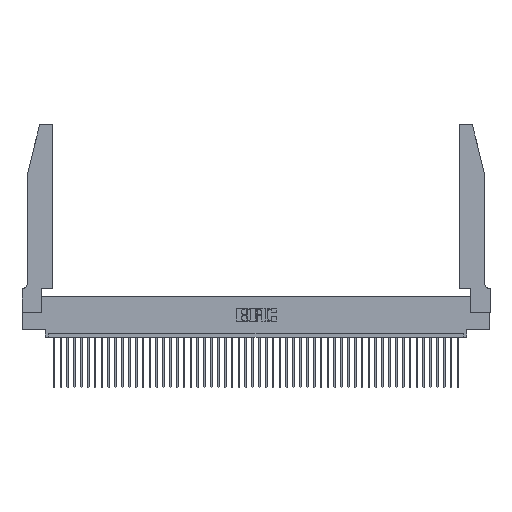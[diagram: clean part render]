
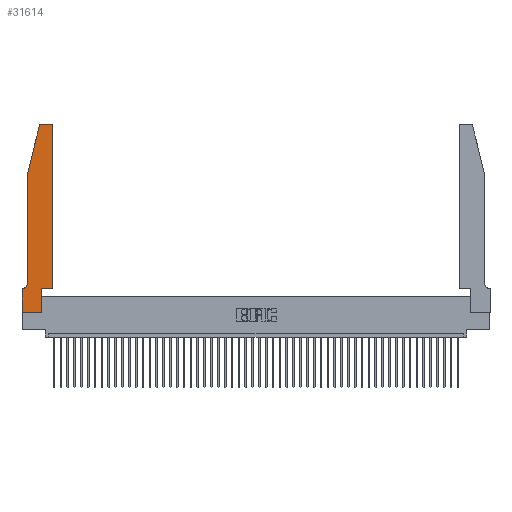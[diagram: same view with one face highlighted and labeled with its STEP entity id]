
A CAD part, top view. The second image highlights one B-rep face of the part: STEP entity #31614.
In plain terms, the highlighted planar face has unit normal (0, 0, 1).
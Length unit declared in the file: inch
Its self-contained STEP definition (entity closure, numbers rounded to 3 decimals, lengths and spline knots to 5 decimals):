
#849 = LINE ( 'NONE', #23890, #14673 ) ;
#1057 = VERTEX_POINT ( 'NONE', #4932 ) ;
#1061 = ORIENTED_EDGE ( 'NONE', *, *, #10899, .T. ) ;
#1117 = CARTESIAN_POINT ( 'NONE',  ( 0.2865, 0.35, 0.37 ) ) ;
#1268 = CARTESIAN_POINT ( 'NONE',  ( 0.0055, 0.42, 0.37 ) ) ;
#1487 = CIRCLE ( 'NONE', #10170, 0.03 ) ;
#1803 = EDGE_CURVE ( 'NONE', #27731, #20160, #37161, .T. ) ;
#2335 = ORIENTED_EDGE ( 'NONE', *, *, #33796, .T. ) ;
#2432 = CARTESIAN_POINT ( 'NONE',  ( 0.4205, 2.75, 0.37 ) ) ;
#2512 = DIRECTION ( 'NONE',  ( 1., 0., 0. ) ) ;
#2964 = DIRECTION ( 'NONE',  ( 1., 0., 0. ) ) ;
#2993 = DIRECTION ( 'NONE',  ( 1., 0., 0. ) ) ;
#4932 = CARTESIAN_POINT ( 'NONE',  ( 0.0755, 0.42, 0.37 ) ) ;
#5509 = DIRECTION ( 'NONE',  ( -1., 0., 0. ) ) ;
#5576 = EDGE_CURVE ( 'NONE', #1057, #28764, #26000, .T. ) ;
#5827 = CARTESIAN_POINT ( 'NONE',  ( 0.25487, 2.72718, 0.37 ) ) ;
#6089 = CARTESIAN_POINT ( 'NONE',  ( 0.2865, 0.35, 0.37 ) ) ;
#6396 = CARTESIAN_POINT ( 'NONE',  ( 0.0755, 2., 0.37 ) ) ;
#7284 = EDGE_CURVE ( 'NONE', #18102, #23881, #47215, .T. ) ;
#8671 = DIRECTION ( 'NONE',  ( 0., 0., -1. ) ) ;
#8726 = LINE ( 'NONE', #45973, #35723 ) ;
#8830 = VERTEX_POINT ( 'NONE', #6396 ) ;
#9188 = VECTOR ( 'NONE', #16261, 39.37008 ) ;
#9238 = LINE ( 'NONE', #46732, #40277 ) ;
#9920 = DIRECTION ( 'NONE',  ( 0., 0., 1. ) ) ;
#10170 = AXIS2_PLACEMENT_3D ( 'NONE', #32507, #13901, #2964 ) ;
#10325 = ORIENTED_EDGE ( 'NONE', *, *, #29981, .T. ) ;
#10899 = EDGE_CURVE ( 'NONE', #20160, #36525, #8726, .T. ) ;
#11090 = EDGE_CURVE ( 'NONE', #22170, #18102, #36836, .T. ) ;
#12006 = LINE ( 'NONE', #33722, #9188 ) ;
#12334 = DIRECTION ( 'NONE',  ( -1., 0., 0. ) ) ;
#13901 = DIRECTION ( 'NONE',  ( 0., 0., 1. ) ) ;
#14673 = VECTOR ( 'NONE', #38325, 39.37008 ) ;
#14909 = ORIENTED_EDGE ( 'NONE', *, *, #25732, .T. ) ;
#15076 = VECTOR ( 'NONE', #31652, 39.37008 ) ;
#15883 = DIRECTION ( 'NONE',  ( 0., 1., 0. ) ) ;
#15947 = DIRECTION ( 'NONE',  ( 0., -1., 0. ) ) ;
#16261 = DIRECTION ( 'NONE',  ( -0.239, -0.971, 0. ) ) ;
#17174 = CARTESIAN_POINT ( 'NONE',  ( 0.4505, 0.35, 0.37 ) ) ;
#17850 = VECTOR ( 'NONE', #21042, 39.37008 ) ;
#18102 = VERTEX_POINT ( 'NONE', #6089 ) ;
#19010 = CARTESIAN_POINT ( 'NONE',  ( 0., 0., 0.37 ) ) ;
#20160 = VERTEX_POINT ( 'NONE', #2432 ) ;
#21042 = DIRECTION ( 'NONE',  ( 1., 0., 0. ) ) ;
#21153 = PLANE ( 'NONE',  #25939 ) ;
#22170 = VERTEX_POINT ( 'NONE', #41039 ) ;
#22829 = CARTESIAN_POINT ( 'NONE',  ( 0.4505, 0.35, 0.37 ) ) ;
#23881 = VERTEX_POINT ( 'NONE', #27344 ) ;
#23890 = CARTESIAN_POINT ( 'NONE',  ( 0.0755, 2., 0.37 ) ) ;
#24722 = ORIENTED_EDGE ( 'NONE', *, *, #7284, .T. ) ;
#24850 = LINE ( 'NONE', #27956, #15076 ) ;
#25732 = EDGE_CURVE ( 'NONE', #36525, #34297, #1487, .T. ) ;
#25790 = LINE ( 'NONE', #42960, #39014 ) ;
#25939 = AXIS2_PLACEMENT_3D ( 'NONE', #35602, #36700, #36555 ) ;
#26000 = CIRCLE ( 'NONE', #30926, 0.07 ) ;
#27032 = ORIENTED_EDGE ( 'NONE', *, *, #34434, .T. ) ;
#27344 = CARTESIAN_POINT ( 'NONE',  ( 0.4505, 0.35, 0.37 ) ) ;
#27731 = VERTEX_POINT ( 'NONE', #34540 ) ;
#27747 = CARTESIAN_POINT ( 'NONE',  ( 0.4205, 2.72, 0.37 ) ) ;
#27956 = CARTESIAN_POINT ( 'NONE',  ( 0.0755, 0.35, 0.37 ) ) ;
#28466 = CARTESIAN_POINT ( 'NONE',  ( 0.0055, 0.35, 0.37 ) ) ;
#28764 = VERTEX_POINT ( 'NONE', #28466 ) ;
#29184 = ORIENTED_EDGE ( 'NONE', *, *, #32236, .T. ) ;
#29981 = EDGE_CURVE ( 'NONE', #31408, #22170, #25790, .T. ) ;
#30770 = VECTOR ( 'NONE', #42870, 39.37008 ) ;
#30926 = AXIS2_PLACEMENT_3D ( 'NONE', #1268, #8671, #12334 ) ;
#31045 = CARTESIAN_POINT ( 'NONE',  ( 0.284, 2.75, 0.37 ) ) ;
#31408 = VERTEX_POINT ( 'NONE', #19010 ) ;
#31614 = ADVANCED_FACE ( 'NONE', ( #38837 ), #21153, .T. ) ;
#31652 = DIRECTION ( 'NONE',  ( -1., 0., 0. ) ) ;
#32021 = ORIENTED_EDGE ( 'NONE', *, *, #42389, .T. ) ;
#32236 = EDGE_CURVE ( 'NONE', #8830, #1057, #849, .T. ) ;
#32507 = CARTESIAN_POINT ( 'NONE',  ( 0.284, 2.72, 0.37 ) ) ;
#33722 = CARTESIAN_POINT ( 'NONE',  ( 0.0755, 2., 0.37 ) ) ;
#33796 = EDGE_CURVE ( 'NONE', #44369, #31408, #9238, .T. ) ;
#34297 = VERTEX_POINT ( 'NONE', #5827 ) ;
#34345 = ORIENTED_EDGE ( 'NONE', *, *, #5576, .T. ) ;
#34434 = EDGE_CURVE ( 'NONE', #34297, #8830, #12006, .T. ) ;
#34540 = CARTESIAN_POINT ( 'NONE',  ( 0.4505, 2.72, 0.37 ) ) ;
#35602 = CARTESIAN_POINT ( 'NONE',  ( 0., 0.35, 0.37 ) ) ;
#35723 = VECTOR ( 'NONE', #5509, 39.37008 ) ;
#36525 = VERTEX_POINT ( 'NONE', #31045 ) ;
#36555 = DIRECTION ( 'NONE',  ( 1., 0., 0. ) ) ;
#36656 = EDGE_LOOP ( 'NONE', ( #1061, #14909, #27032, #29184, #34345, #42936, #2335, #10325, #40532, #24722, #32021, #47042 ) ) ;
#36700 = DIRECTION ( 'NONE',  ( 0., 0., 1. ) ) ;
#36836 = LINE ( 'NONE', #1117, #37989 ) ;
#37161 = CIRCLE ( 'NONE', #44340, 0.03 ) ;
#37989 = VECTOR ( 'NONE', #15883, 39.37008 ) ;
#38325 = DIRECTION ( 'NONE',  ( 0., -1., 0. ) ) ;
#38837 = FACE_OUTER_BOUND ( 'NONE', #36656, .T. ) ;
#38958 = EDGE_CURVE ( 'NONE', #28764, #44369, #24850, .T. ) ;
#39014 = VECTOR ( 'NONE', #2993, 39.37008 ) ;
#40277 = VECTOR ( 'NONE', #15947, 39.37008 ) ;
#40532 = ORIENTED_EDGE ( 'NONE', *, *, #11090, .T. ) ;
#41039 = CARTESIAN_POINT ( 'NONE',  ( 0.2865, 0., 0.37 ) ) ;
#42389 = EDGE_CURVE ( 'NONE', #23881, #27731, #46351, .T. ) ;
#42870 = DIRECTION ( 'NONE',  ( 0., 1., 0. ) ) ;
#42936 = ORIENTED_EDGE ( 'NONE', *, *, #38958, .T. ) ;
#42960 = CARTESIAN_POINT ( 'NONE',  ( 0., 0., 0.37 ) ) ;
#44340 = AXIS2_PLACEMENT_3D ( 'NONE', #27747, #9920, #2512 ) ;
#44369 = VERTEX_POINT ( 'NONE', #47361 ) ;
#45973 = CARTESIAN_POINT ( 'NONE',  ( 0.2605, 2.75, 0.37 ) ) ;
#46351 = LINE ( 'NONE', #17174, #30770 ) ;
#46732 = CARTESIAN_POINT ( 'NONE',  ( 0., 0., 0.37 ) ) ;
#47042 = ORIENTED_EDGE ( 'NONE', *, *, #1803, .T. ) ;
#47215 = LINE ( 'NONE', #22829, #17850 ) ;
#47361 = CARTESIAN_POINT ( 'NONE',  ( 0., 0.35, 0.37 ) ) ;
